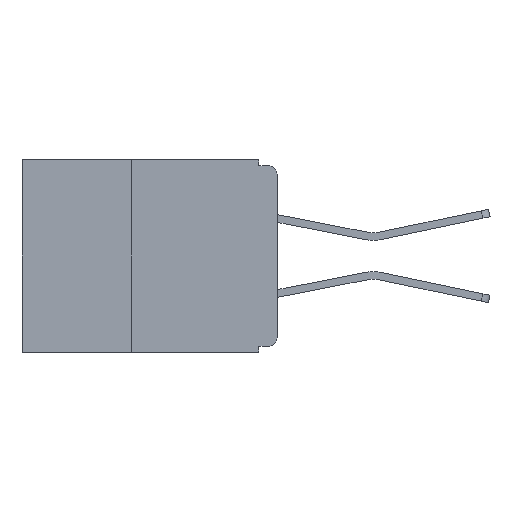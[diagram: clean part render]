
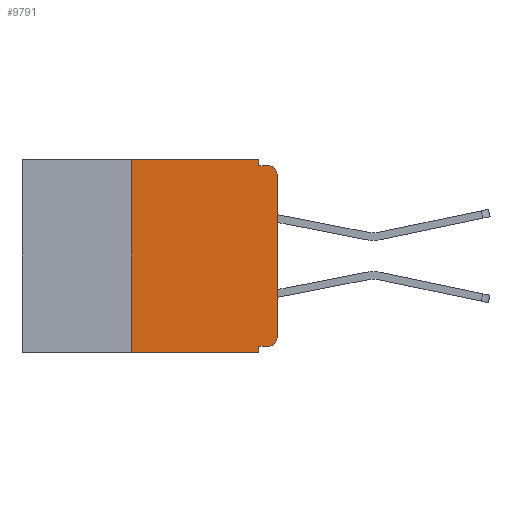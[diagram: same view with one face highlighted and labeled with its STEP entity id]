
A CAD part, left-side view. The second image highlights one B-rep face of the part: STEP entity #9791.
In plain terms, the highlighted planar face has unit normal (-1, 0, 0).
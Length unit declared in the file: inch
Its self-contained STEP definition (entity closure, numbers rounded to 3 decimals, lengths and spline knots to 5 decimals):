
#284 = EDGE_CURVE ( 'NONE', #13548, #18424, #17633, .T. ) ;
#547 = CARTESIAN_POINT ( 'NONE',  ( 0., 0.031, -0.01 ) ) ;
#592 = CARTESIAN_POINT ( 'NONE',  ( 0., 0.031, -0.33 ) ) ;
#840 = VECTOR ( 'NONE', #14425, 39.37008 ) ;
#1153 = PLANE ( 'NONE',  #22898 ) ;
#1189 = LINE ( 'NONE', #22920, #7212 ) ;
#1372 = VERTEX_POINT ( 'NONE', #9073 ) ;
#1682 = CARTESIAN_POINT ( 'NONE',  ( 0., 0.031, 0. ) ) ;
#1717 = CARTESIAN_POINT ( 'NONE',  ( 0., 0.015, -0.025 ) ) ;
#2520 = DIRECTION ( 'NONE',  ( 0., 0., 1. ) ) ;
#2719 = EDGE_CURVE ( 'NONE', #11817, #11976, #7954, .T. ) ;
#2786 = EDGE_CURVE ( 'NONE', #18633, #18424, #18150, .T. ) ;
#2949 = VERTEX_POINT ( 'NONE', #1682 ) ;
#3111 = CARTESIAN_POINT ( 'NONE',  ( 0., 0.25, -0.33 ) ) ;
#3112 = EDGE_CURVE ( 'NONE', #1372, #12443, #4408, .T. ) ;
#3156 = DIRECTION ( 'NONE',  ( 0., 0., -1. ) ) ;
#4235 = EDGE_CURVE ( 'NONE', #12443, #11817, #5301, .T. ) ;
#4408 = CIRCLE ( 'NONE', #10680, 0.015 ) ;
#4515 = DIRECTION ( 'NONE',  ( -1., 0., 0. ) ) ;
#4583 = DIRECTION ( 'NONE',  ( 0., 0., -1. ) ) ;
#4633 = EDGE_CURVE ( 'NONE', #12808, #11976, #1189, .T. ) ;
#5283 = CARTESIAN_POINT ( 'NONE',  ( 0., 0.031, -0.32 ) ) ;
#5301 = LINE ( 'NONE', #15459, #18074 ) ;
#5323 = EDGE_CURVE ( 'NONE', #18633, #17692, #6012, .T. ) ;
#5486 = DIRECTION ( 'NONE',  ( 0., 0., -1. ) ) ;
#5494 = VECTOR ( 'NONE', #25795, 39.37008 ) ;
#6012 = LINE ( 'NONE', #3111, #16230 ) ;
#6177 = ORIENTED_EDGE ( 'NONE', *, *, #9254, .F. ) ;
#7063 = VECTOR ( 'NONE', #5486, 39.37008 ) ;
#7212 = VECTOR ( 'NONE', #22887, 39.37008 ) ;
#7494 = ORIENTED_EDGE ( 'NONE', *, *, #4633, .F. ) ;
#7707 = LINE ( 'NONE', #17712, #7063 ) ;
#7954 = CIRCLE ( 'NONE', #25295, 0.015 ) ;
#9073 = CARTESIAN_POINT ( 'NONE',  ( 0., 0.015, -0.32 ) ) ;
#9254 = EDGE_CURVE ( 'NONE', #2949, #12808, #7707, .T. ) ;
#9455 = CARTESIAN_POINT ( 'NONE',  ( 0., 0.437, -0.33 ) ) ;
#9468 = EDGE_LOOP ( 'NONE', ( #18038, #20423, #7494, #6177, #25820, #16755, #18347, #11693, #21967, #21014 ) ) ;
#9635 = CARTESIAN_POINT ( 'NONE',  ( 0., 0., -0.305 ) ) ;
#9791 = ADVANCED_FACE ( 'NONE', ( #21387 ), #1153, .F. ) ;
#10292 = CARTESIAN_POINT ( 'NONE',  ( 0., 0., -0.32 ) ) ;
#10680 = AXIS2_PLACEMENT_3D ( 'NONE', #21823, #19638, #19577 ) ;
#11693 = ORIENTED_EDGE ( 'NONE', *, *, #284, .F. ) ;
#11817 = VERTEX_POINT ( 'NONE', #17861 ) ;
#11976 = VERTEX_POINT ( 'NONE', #24410 ) ;
#12443 = VERTEX_POINT ( 'NONE', #9635 ) ;
#12808 = VERTEX_POINT ( 'NONE', #547 ) ;
#13054 = EDGE_CURVE ( 'NONE', #17692, #2949, #21253, .T. ) ;
#13548 = VERTEX_POINT ( 'NONE', #5283 ) ;
#13838 = EDGE_CURVE ( 'NONE', #1372, #13548, #17080, .T. ) ;
#14425 = DIRECTION ( 'NONE',  ( 0., 1., 0. ) ) ;
#15234 = DIRECTION ( 'NONE',  ( 0., 0., 1. ) ) ;
#15240 = VECTOR ( 'NONE', #25669, 39.37008 ) ;
#15407 = DIRECTION ( 'NONE',  ( 1., 0., 0. ) ) ;
#15459 = CARTESIAN_POINT ( 'NONE',  ( 0., 0., 0. ) ) ;
#15511 = DIRECTION ( 'NONE',  ( 0., -1., 0. ) ) ;
#16230 = VECTOR ( 'NONE', #2520, 39.37008 ) ;
#16755 = ORIENTED_EDGE ( 'NONE', *, *, #5323, .F. ) ;
#16792 = CARTESIAN_POINT ( 'NONE',  ( 0., 0.25, -0.33 ) ) ;
#17080 = LINE ( 'NONE', #10292, #840 ) ;
#17358 = CARTESIAN_POINT ( 'NONE',  ( 0., 0.25, 0. ) ) ;
#17633 = LINE ( 'NONE', #592, #5494 ) ;
#17692 = VERTEX_POINT ( 'NONE', #17358 ) ;
#17712 = CARTESIAN_POINT ( 'NONE',  ( 0., 0.031, 0. ) ) ;
#17861 = CARTESIAN_POINT ( 'NONE',  ( 0., 0., -0.025 ) ) ;
#18038 = ORIENTED_EDGE ( 'NONE', *, *, #4235, .T. ) ;
#18074 = VECTOR ( 'NONE', #15234, 39.37008 ) ;
#18150 = LINE ( 'NONE', #9455, #22270 ) ;
#18347 = ORIENTED_EDGE ( 'NONE', *, *, #2786, .T. ) ;
#18424 = VERTEX_POINT ( 'NONE', #24338 ) ;
#18633 = VERTEX_POINT ( 'NONE', #16792 ) ;
#19577 = DIRECTION ( 'NONE',  ( 0., 0., -1. ) ) ;
#19638 = DIRECTION ( 'NONE',  ( -1., 0., 0. ) ) ;
#20423 = ORIENTED_EDGE ( 'NONE', *, *, #2719, .T. ) ;
#21014 = ORIENTED_EDGE ( 'NONE', *, *, #3112, .T. ) ;
#21253 = LINE ( 'NONE', #21617, #15240 ) ;
#21387 = FACE_OUTER_BOUND ( 'NONE', #9468, .T. ) ;
#21617 = CARTESIAN_POINT ( 'NONE',  ( 0., 0.437, 0. ) ) ;
#21823 = CARTESIAN_POINT ( 'NONE',  ( 0., 0.015, -0.305 ) ) ;
#21967 = ORIENTED_EDGE ( 'NONE', *, *, #13838, .F. ) ;
#22270 = VECTOR ( 'NONE', #15511, 39.37008 ) ;
#22887 = DIRECTION ( 'NONE',  ( 0., -1., 0. ) ) ;
#22898 = AXIS2_PLACEMENT_3D ( 'NONE', #25477, #15407, #3156 ) ;
#22920 = CARTESIAN_POINT ( 'NONE',  ( 0., 0., -0.01 ) ) ;
#24338 = CARTESIAN_POINT ( 'NONE',  ( 0., 0.031, -0.33 ) ) ;
#24410 = CARTESIAN_POINT ( 'NONE',  ( 0., 0.015, -0.01 ) ) ;
#25295 = AXIS2_PLACEMENT_3D ( 'NONE', #1717, #4515, #4583 ) ;
#25477 = CARTESIAN_POINT ( 'NONE',  ( 0., 0.437, 0. ) ) ;
#25669 = DIRECTION ( 'NONE',  ( 0., -1., 0. ) ) ;
#25795 = DIRECTION ( 'NONE',  ( 0., 0., -1. ) ) ;
#25820 = ORIENTED_EDGE ( 'NONE', *, *, #13054, .F. ) ;
